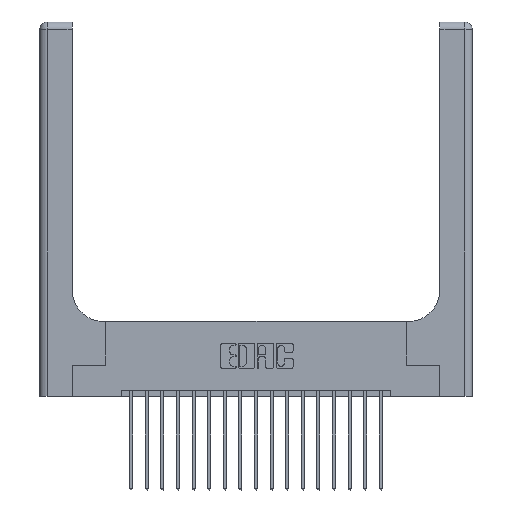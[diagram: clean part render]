
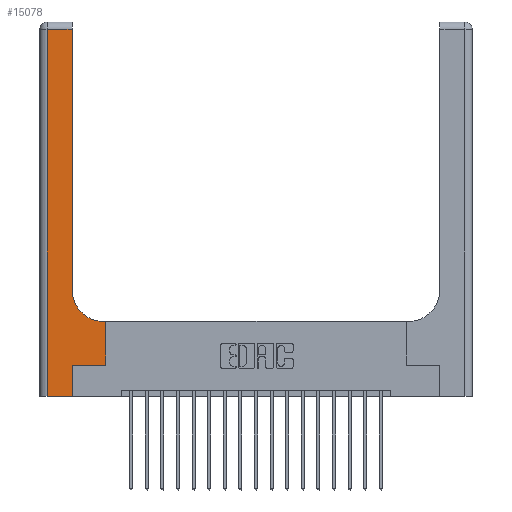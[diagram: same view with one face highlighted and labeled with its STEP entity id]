
A CAD part, top view. The second image highlights one B-rep face of the part: STEP entity #15078.
In plain terms, the highlighted planar face has unit normal (0, 0, 1).
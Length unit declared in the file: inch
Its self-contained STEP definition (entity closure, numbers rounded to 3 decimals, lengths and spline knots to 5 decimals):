
#116 = VECTOR ( 'NONE', #19792, 39.37008 ) ;
#837 = VERTEX_POINT ( 'NONE', #9554 ) ;
#2156 = CARTESIAN_POINT ( 'NONE',  ( 0., 2.94, 0.37 ) ) ;
#2294 = ORIENTED_EDGE ( 'NONE', *, *, #2365, .T. ) ;
#2365 = EDGE_CURVE ( 'NONE', #12938, #16938, #18671, .T. ) ;
#2441 = DIRECTION ( 'NONE',  ( 1., 0., 0. ) ) ;
#2546 = VECTOR ( 'NONE', #2441, 39.37008 ) ;
#2636 = DIRECTION ( 'NONE',  ( 1., 0., 0. ) ) ;
#2995 = EDGE_CURVE ( 'NONE', #15576, #4152, #9466, .T. ) ;
#3211 = VECTOR ( 'NONE', #14118, 39.37008 ) ;
#3520 = LINE ( 'NONE', #15932, #9697 ) ;
#3646 = FACE_OUTER_BOUND ( 'NONE', #5726, .T. ) ;
#3705 = ORIENTED_EDGE ( 'NONE', *, *, #5334, .T. ) ;
#3788 = CARTESIAN_POINT ( 'NONE',  ( 0.26, 0.6, 0.37 ) ) ;
#3885 = VECTOR ( 'NONE', #5540, 39.37008 ) ;
#4079 = CARTESIAN_POINT ( 'NONE',  ( 0.265, 0., 0.37 ) ) ;
#4123 = AXIS2_PLACEMENT_3D ( 'NONE', #8746, #14930, #19291 ) ;
#4152 = VERTEX_POINT ( 'NONE', #9771 ) ;
#4555 = EDGE_CURVE ( 'NONE', #16706, #12097, #8811, .T. ) ;
#4858 = ORIENTED_EDGE ( 'NONE', *, *, #5895, .T. ) ;
#4909 = ORIENTED_EDGE ( 'NONE', *, *, #17456, .T. ) ;
#5036 = DIRECTION ( 'NONE',  ( -1., 0., 0. ) ) ;
#5176 = ORIENTED_EDGE ( 'NONE', *, *, #10656, .T. ) ;
#5334 = EDGE_CURVE ( 'NONE', #837, #12938, #18959, .T. ) ;
#5540 = DIRECTION ( 'NONE',  ( -1., 0., 0. ) ) ;
#5726 = EDGE_LOOP ( 'NONE', ( #5176, #3705, #2294, #4909, #17341, #4858, #13382, #11339, #15133 ) ) ;
#5808 = VERTEX_POINT ( 'NONE', #4079 ) ;
#5895 = EDGE_CURVE ( 'NONE', #13497, #15576, #13357, .T. ) ;
#7630 = CARTESIAN_POINT ( 'NONE',  ( 0., 0., 0.37 ) ) ;
#8214 = DIRECTION ( 'NONE',  ( 0., 1., 0. ) ) ;
#8746 = CARTESIAN_POINT ( 'NONE',  ( 0., 3., 0.37 ) ) ;
#8811 = CIRCLE ( 'NONE', #14298, 0.25 ) ;
#9013 = CARTESIAN_POINT ( 'NONE',  ( 0.06, 0., 0.37 ) ) ;
#9268 = CARTESIAN_POINT ( 'NONE',  ( 0.265, 0., 0.37 ) ) ;
#9466 = LINE ( 'NONE', #15663, #11039 ) ;
#9554 = CARTESIAN_POINT ( 'NONE',  ( 0.26, 2.94, 0.37 ) ) ;
#9558 = LINE ( 'NONE', #7630, #3211 ) ;
#9697 = VECTOR ( 'NONE', #8214, 39.37008 ) ;
#9771 = CARTESIAN_POINT ( 'NONE',  ( 0.528, 0.6, 0.37 ) ) ;
#9859 = PLANE ( 'NONE',  #4123 ) ;
#10319 = LINE ( 'NONE', #9268, #16483 ) ;
#10656 = EDGE_CURVE ( 'NONE', #12097, #837, #3520, .T. ) ;
#10997 = EDGE_CURVE ( 'NONE', #4152, #16706, #17728, .T. ) ;
#11039 = VECTOR ( 'NONE', #14125, 39.37008 ) ;
#11339 = ORIENTED_EDGE ( 'NONE', *, *, #10997, .T. ) ;
#11488 = CARTESIAN_POINT ( 'NONE',  ( 0.265, 0.25, 0.37 ) ) ;
#12097 = VERTEX_POINT ( 'NONE', #17731 ) ;
#12301 = CARTESIAN_POINT ( 'NONE',  ( 0.06, 3., 0.37 ) ) ;
#12938 = VERTEX_POINT ( 'NONE', #18908 ) ;
#13357 = LINE ( 'NONE', #13639, #2546 ) ;
#13382 = ORIENTED_EDGE ( 'NONE', *, *, #2995, .T. ) ;
#13497 = VERTEX_POINT ( 'NONE', #11488 ) ;
#13639 = CARTESIAN_POINT ( 'NONE',  ( 0.265, 0.25, 0.37 ) ) ;
#14017 = EDGE_CURVE ( 'NONE', #5808, #13497, #10319, .T. ) ;
#14118 = DIRECTION ( 'NONE',  ( 1., 0., 0. ) ) ;
#14125 = DIRECTION ( 'NONE',  ( 0., 1., 0. ) ) ;
#14298 = AXIS2_PLACEMENT_3D ( 'NONE', #19608, #18296, #2636 ) ;
#14930 = DIRECTION ( 'NONE',  ( 0., 0., -1. ) ) ;
#15078 = ADVANCED_FACE ( 'NONE', ( #3646 ), #9859, .F. ) ;
#15133 = ORIENTED_EDGE ( 'NONE', *, *, #4555, .T. ) ;
#15228 = VECTOR ( 'NONE', #5036, 39.37008 ) ;
#15576 = VERTEX_POINT ( 'NONE', #18223 ) ;
#15663 = CARTESIAN_POINT ( 'NONE',  ( 0.528, 0.25, 0.37 ) ) ;
#15932 = CARTESIAN_POINT ( 'NONE',  ( 0.26, 3., 0.37 ) ) ;
#16327 = CARTESIAN_POINT ( 'NONE',  ( 0.51, 0.6, 0.37 ) ) ;
#16483 = VECTOR ( 'NONE', #16505, 39.37008 ) ;
#16505 = DIRECTION ( 'NONE',  ( 0., 1., 0. ) ) ;
#16706 = VERTEX_POINT ( 'NONE', #16327 ) ;
#16938 = VERTEX_POINT ( 'NONE', #9013 ) ;
#17341 = ORIENTED_EDGE ( 'NONE', *, *, #14017, .T. ) ;
#17456 = EDGE_CURVE ( 'NONE', #16938, #5808, #9558, .T. ) ;
#17728 = LINE ( 'NONE', #3788, #3885 ) ;
#17731 = CARTESIAN_POINT ( 'NONE',  ( 0.26, 0.85, 0.37 ) ) ;
#18223 = CARTESIAN_POINT ( 'NONE',  ( 0.528, 0.25, 0.37 ) ) ;
#18296 = DIRECTION ( 'NONE',  ( 0., 0., -1. ) ) ;
#18671 = LINE ( 'NONE', #12301, #116 ) ;
#18908 = CARTESIAN_POINT ( 'NONE',  ( 0.06, 2.94, 0.37 ) ) ;
#18959 = LINE ( 'NONE', #2156, #15228 ) ;
#19291 = DIRECTION ( 'NONE',  ( -1., 0., 0. ) ) ;
#19608 = CARTESIAN_POINT ( 'NONE',  ( 0.51, 0.85, 0.37 ) ) ;
#19792 = DIRECTION ( 'NONE',  ( 0., -1., 0. ) ) ;
